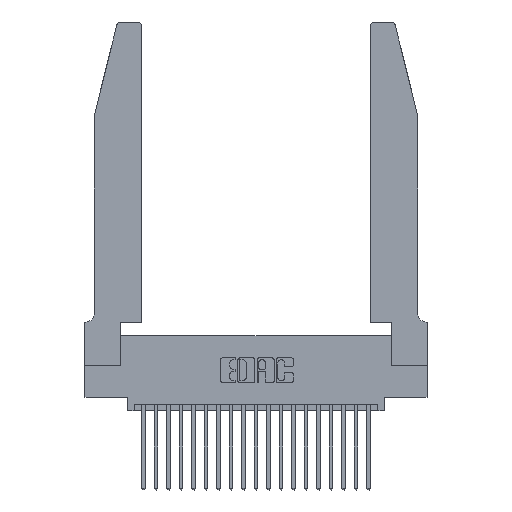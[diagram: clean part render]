
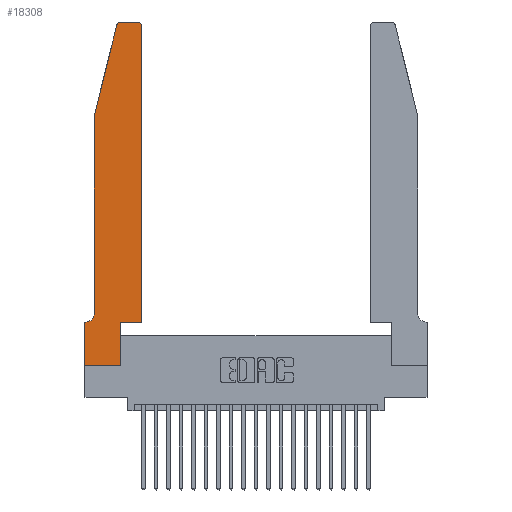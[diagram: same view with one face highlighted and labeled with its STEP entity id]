
A CAD part, top view. The second image highlights one B-rep face of the part: STEP entity #18308.
In plain terms, the highlighted planar face has unit normal (0, 0, 1).
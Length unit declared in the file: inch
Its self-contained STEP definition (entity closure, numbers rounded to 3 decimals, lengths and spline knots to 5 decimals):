
#117 = EDGE_CURVE ( 'NONE', #9772, #9904, #10162, .T. ) ;
#254 = CARTESIAN_POINT ( 'NONE',  ( 0.4505, 2.72, 0.37 ) ) ;
#297 = VECTOR ( 'NONE', #1825, 39.37008 ) ;
#312 = AXIS2_PLACEMENT_3D ( 'NONE', #10577, #20762, #20062 ) ;
#502 = VERTEX_POINT ( 'NONE', #1107 ) ;
#1100 = EDGE_CURVE ( 'NONE', #22857, #10789, #1356, .T. ) ;
#1107 = CARTESIAN_POINT ( 'NONE',  ( 0., 0., 0.37 ) ) ;
#1356 = CIRCLE ( 'NONE', #12777, 0.03 ) ;
#1462 = ORIENTED_EDGE ( 'NONE', *, *, #1922, .T. ) ;
#1494 = PLANE ( 'NONE',  #7607 ) ;
#1707 = DIRECTION ( 'NONE',  ( 0., 1., 0. ) ) ;
#1825 = DIRECTION ( 'NONE',  ( -1., 0., 0. ) ) ;
#1922 = EDGE_CURVE ( 'NONE', #7292, #4933, #19002, .T. ) ;
#3038 = ORIENTED_EDGE ( 'NONE', *, *, #3709, .T. ) ;
#3389 = DIRECTION ( 'NONE',  ( 1., 0., 0. ) ) ;
#3431 = LINE ( 'NONE', #11135, #16486 ) ;
#3709 = EDGE_CURVE ( 'NONE', #502, #14564, #19191, .T. ) ;
#3894 = ORIENTED_EDGE ( 'NONE', *, *, #17211, .T. ) ;
#3985 = ORIENTED_EDGE ( 'NONE', *, *, #18836, .T. ) ;
#4933 = VERTEX_POINT ( 'NONE', #22843 ) ;
#5703 = VECTOR ( 'NONE', #16795, 39.37008 ) ;
#5817 = DIRECTION ( 'NONE',  ( 0., 1., 0. ) ) ;
#6072 = CARTESIAN_POINT ( 'NONE',  ( 0.2865, 0., 0.37 ) ) ;
#6202 = CARTESIAN_POINT ( 'NONE',  ( 0., 0., 0.37 ) ) ;
#6230 = DIRECTION ( 'NONE',  ( -1., 0., 0. ) ) ;
#6966 = VECTOR ( 'NONE', #21358, 39.37008 ) ;
#7017 = EDGE_CURVE ( 'NONE', #10789, #17267, #12301, .T. ) ;
#7284 = DIRECTION ( 'NONE',  ( 0., 0., -1. ) ) ;
#7292 = VERTEX_POINT ( 'NONE', #17509 ) ;
#7442 = CARTESIAN_POINT ( 'NONE',  ( 0.0755, 2., 0.37 ) ) ;
#7607 = AXIS2_PLACEMENT_3D ( 'NONE', #20921, #14088, #3389 ) ;
#7655 = ORIENTED_EDGE ( 'NONE', *, *, #10304, .T. ) ;
#7962 = ORIENTED_EDGE ( 'NONE', *, *, #117, .T. ) ;
#7965 = ORIENTED_EDGE ( 'NONE', *, *, #10417, .T. ) ;
#8096 = DIRECTION ( 'NONE',  ( -0.239, -0.971, 0. ) ) ;
#8558 = DIRECTION ( 'NONE',  ( 0., 0., 1. ) ) ;
#9110 = VECTOR ( 'NONE', #19697, 39.37008 ) ;
#9206 = CARTESIAN_POINT ( 'NONE',  ( 0.0755, 2., 0.37 ) ) ;
#9378 = EDGE_CURVE ( 'NONE', #9904, #22857, #13607, .T. ) ;
#9772 = VERTEX_POINT ( 'NONE', #254 ) ;
#9904 = VERTEX_POINT ( 'NONE', #21866 ) ;
#10162 = CIRCLE ( 'NONE', #312, 0.03 ) ;
#10266 = VECTOR ( 'NONE', #21722, 39.37008 ) ;
#10304 = EDGE_CURVE ( 'NONE', #14564, #7292, #20539, .T. ) ;
#10417 = EDGE_CURVE ( 'NONE', #15997, #502, #22929, .T. ) ;
#10577 = CARTESIAN_POINT ( 'NONE',  ( 0.4205, 2.72, 0.37 ) ) ;
#10737 = CARTESIAN_POINT ( 'NONE',  ( 0.284, 2.72, 0.37 ) ) ;
#10789 = VERTEX_POINT ( 'NONE', #18784 ) ;
#11029 = CARTESIAN_POINT ( 'NONE',  ( 0., 0., 0.37 ) ) ;
#11135 = CARTESIAN_POINT ( 'NONE',  ( 0.4505, 0.35, 0.37 ) ) ;
#11684 = FACE_OUTER_BOUND ( 'NONE', #16981, .T. ) ;
#11755 = VECTOR ( 'NONE', #8096, 39.37008 ) ;
#11993 = CARTESIAN_POINT ( 'NONE',  ( 0.284, 2.75, 0.37 ) ) ;
#12301 = LINE ( 'NONE', #22001, #11755 ) ;
#12577 = ORIENTED_EDGE ( 'NONE', *, *, #16665, .T. ) ;
#12777 = AXIS2_PLACEMENT_3D ( 'NONE', #10737, #8558, #13841 ) ;
#13056 = ORIENTED_EDGE ( 'NONE', *, *, #1100, .T. ) ;
#13177 = CARTESIAN_POINT ( 'NONE',  ( 0.4505, 0.35, 0.37 ) ) ;
#13607 = LINE ( 'NONE', #18556, #21648 ) ;
#13841 = DIRECTION ( 'NONE',  ( 1., 0., 0. ) ) ;
#14004 = VERTEX_POINT ( 'NONE', #18646 ) ;
#14088 = DIRECTION ( 'NONE',  ( 0., 0., 1. ) ) ;
#14149 = AXIS2_PLACEMENT_3D ( 'NONE', #17828, #7284, #19551 ) ;
#14322 = ORIENTED_EDGE ( 'NONE', *, *, #7017, .T. ) ;
#14564 = VERTEX_POINT ( 'NONE', #6072 ) ;
#15231 = LINE ( 'NONE', #22856, #297 ) ;
#15983 = VECTOR ( 'NONE', #1707, 39.37008 ) ;
#15997 = VERTEX_POINT ( 'NONE', #17949 ) ;
#16486 = VECTOR ( 'NONE', #5817, 39.37008 ) ;
#16665 = EDGE_CURVE ( 'NONE', #17267, #22118, #20385, .T. ) ;
#16795 = DIRECTION ( 'NONE',  ( 1., 0., 0. ) ) ;
#16981 = EDGE_LOOP ( 'NONE', ( #17651, #13056, #14322, #12577, #3894, #3985, #7965, #3038, #7655, #1462, #20251, #7962 ) ) ;
#17211 = EDGE_CURVE ( 'NONE', #22118, #14004, #19608, .T. ) ;
#17267 = VERTEX_POINT ( 'NONE', #7442 ) ;
#17509 = CARTESIAN_POINT ( 'NONE',  ( 0.2865, 0.35, 0.37 ) ) ;
#17651 = ORIENTED_EDGE ( 'NONE', *, *, #9378, .T. ) ;
#17828 = CARTESIAN_POINT ( 'NONE',  ( 0.0055, 0.42, 0.37 ) ) ;
#17949 = CARTESIAN_POINT ( 'NONE',  ( 0., 0.35, 0.37 ) ) ;
#18308 = ADVANCED_FACE ( 'NONE', ( #11684 ), #1494, .T. ) ;
#18556 = CARTESIAN_POINT ( 'NONE',  ( 0.2605, 2.75, 0.37 ) ) ;
#18646 = CARTESIAN_POINT ( 'NONE',  ( 0.0055, 0.35, 0.37 ) ) ;
#18784 = CARTESIAN_POINT ( 'NONE',  ( 0.25487, 2.72718, 0.37 ) ) ;
#18836 = EDGE_CURVE ( 'NONE', #14004, #15997, #15231, .T. ) ;
#19002 = LINE ( 'NONE', #13177, #10266 ) ;
#19191 = LINE ( 'NONE', #6202, #5703 ) ;
#19551 = DIRECTION ( 'NONE',  ( -1., 0., 0. ) ) ;
#19608 = CIRCLE ( 'NONE', #14149, 0.07 ) ;
#19697 = DIRECTION ( 'NONE',  ( 0., -1., 0. ) ) ;
#20061 = CARTESIAN_POINT ( 'NONE',  ( 0.0755, 0.42, 0.37 ) ) ;
#20062 = DIRECTION ( 'NONE',  ( 1., 0., 0. ) ) ;
#20251 = ORIENTED_EDGE ( 'NONE', *, *, #20828, .T. ) ;
#20385 = LINE ( 'NONE', #9206, #6966 ) ;
#20539 = LINE ( 'NONE', #22816, #15983 ) ;
#20762 = DIRECTION ( 'NONE',  ( 0., 0., 1. ) ) ;
#20828 = EDGE_CURVE ( 'NONE', #4933, #9772, #3431, .T. ) ;
#20921 = CARTESIAN_POINT ( 'NONE',  ( 0., 0.35, 0.37 ) ) ;
#21358 = DIRECTION ( 'NONE',  ( 0., -1., 0. ) ) ;
#21648 = VECTOR ( 'NONE', #6230, 39.37008 ) ;
#21722 = DIRECTION ( 'NONE',  ( 1., 0., 0. ) ) ;
#21866 = CARTESIAN_POINT ( 'NONE',  ( 0.4205, 2.75, 0.37 ) ) ;
#22001 = CARTESIAN_POINT ( 'NONE',  ( 0.0755, 2., 0.37 ) ) ;
#22118 = VERTEX_POINT ( 'NONE', #20061 ) ;
#22816 = CARTESIAN_POINT ( 'NONE',  ( 0.2865, 0.35, 0.37 ) ) ;
#22843 = CARTESIAN_POINT ( 'NONE',  ( 0.4505, 0.35, 0.37 ) ) ;
#22856 = CARTESIAN_POINT ( 'NONE',  ( 0.0755, 0.35, 0.37 ) ) ;
#22857 = VERTEX_POINT ( 'NONE', #11993 ) ;
#22929 = LINE ( 'NONE', #11029, #9110 ) ;
